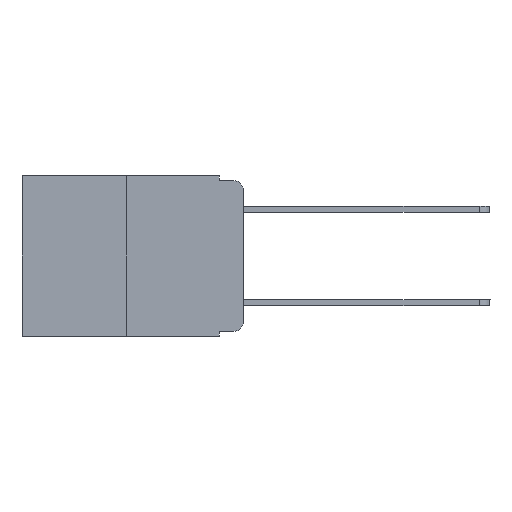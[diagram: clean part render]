
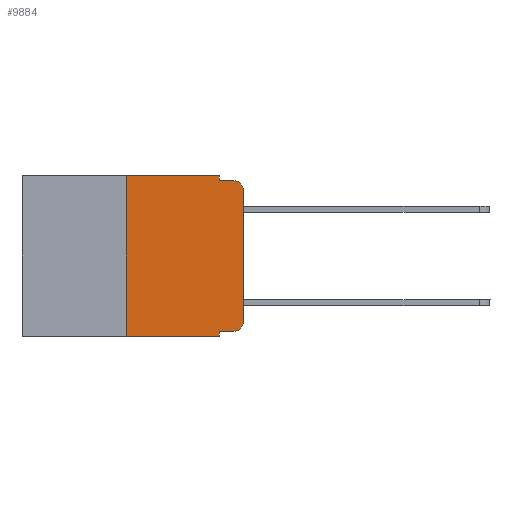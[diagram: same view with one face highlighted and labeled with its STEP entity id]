
A CAD part, left-side view. The second image highlights one B-rep face of the part: STEP entity #9884.
In plain terms, the highlighted planar face has unit normal (-1, 0, 0).
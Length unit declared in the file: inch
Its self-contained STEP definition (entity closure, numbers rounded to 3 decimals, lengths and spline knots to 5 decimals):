
#197 = DIRECTION ( 'NONE',  ( 0., -1., 0. ) ) ;
#403 = LINE ( 'NONE', #5945, #8011 ) ;
#513 = DIRECTION ( 'NONE',  ( 0., -1., 0. ) ) ;
#864 = VERTEX_POINT ( 'NONE', #8967 ) ;
#872 = EDGE_LOOP ( 'NONE', ( #10765, #11012, #3093, #997, #9420, #1775, #10407, #6484, #1513, #9154 ) ) ;
#997 = ORIENTED_EDGE ( 'NONE', *, *, #5999, .F. ) ;
#1007 = CARTESIAN_POINT ( 'NONE',  ( 0., 0.473, 0. ) ) ;
#1102 = EDGE_CURVE ( 'NONE', #2378, #2417, #6632, .T. ) ;
#1237 = CARTESIAN_POINT ( 'NONE',  ( 0., 0.25, -0.343 ) ) ;
#1356 = CARTESIAN_POINT ( 'NONE',  ( 0., 0.473, -0.343 ) ) ;
#1513 = ORIENTED_EDGE ( 'NONE', *, *, #3057, .T. ) ;
#1562 = DIRECTION ( 'NONE',  ( -1., 0., 0. ) ) ;
#1775 = ORIENTED_EDGE ( 'NONE', *, *, #5760, .F. ) ;
#1803 = CARTESIAN_POINT ( 'NONE',  ( 0., 0., -0.313 ) ) ;
#2030 = CARTESIAN_POINT ( 'NONE',  ( 0., 0., 0. ) ) ;
#2205 = EDGE_CURVE ( 'NONE', #4691, #2378, #4605, .T. ) ;
#2235 = VERTEX_POINT ( 'NONE', #1237 ) ;
#2378 = VERTEX_POINT ( 'NONE', #6835 ) ;
#2417 = VERTEX_POINT ( 'NONE', #5220 ) ;
#2481 = DIRECTION ( 'NONE',  ( 0., 0., -1. ) ) ;
#2568 = EDGE_CURVE ( 'NONE', #10823, #3773, #5002, .T. ) ;
#2684 = DIRECTION ( 'NONE',  ( 1., 0., 0. ) ) ;
#2881 = VECTOR ( 'NONE', #8968, 39.37008 ) ;
#2986 = CARTESIAN_POINT ( 'NONE',  ( 0., 0.051, -0.333 ) ) ;
#3057 = EDGE_CURVE ( 'NONE', #10823, #3672, #9598, .T. ) ;
#3093 = ORIENTED_EDGE ( 'NONE', *, *, #5106, .F. ) ;
#3416 = DIRECTION ( 'NONE',  ( 0., 0., -1. ) ) ;
#3422 = FACE_OUTER_BOUND ( 'NONE', #872, .T. ) ;
#3605 = AXIS2_PLACEMENT_3D ( 'NONE', #7185, #4580, #6220 ) ;
#3672 = VERTEX_POINT ( 'NONE', #8116 ) ;
#3773 = VERTEX_POINT ( 'NONE', #4777 ) ;
#4003 = LINE ( 'NONE', #4593, #4669 ) ;
#4103 = DIRECTION ( 'NONE',  ( 0., 0., 1. ) ) ;
#4577 = CARTESIAN_POINT ( 'NONE',  ( 0., 0.25, 0. ) ) ;
#4580 = DIRECTION ( 'NONE',  ( -1., 0., 0. ) ) ;
#4593 = CARTESIAN_POINT ( 'NONE',  ( 0., 0.051, -0.01 ) ) ;
#4605 = LINE ( 'NONE', #2030, #2881 ) ;
#4624 = CARTESIAN_POINT ( 'NONE',  ( 0., 0.051, -0.333 ) ) ;
#4669 = VECTOR ( 'NONE', #8872, 39.37008 ) ;
#4691 = VERTEX_POINT ( 'NONE', #1803 ) ;
#4745 = VECTOR ( 'NONE', #9021, 39.37008 ) ;
#4777 = CARTESIAN_POINT ( 'NONE',  ( 0., 0.051, -0.343 ) ) ;
#5002 = LINE ( 'NONE', #10677, #4745 ) ;
#5106 = EDGE_CURVE ( 'NONE', #864, #2417, #4003, .T. ) ;
#5220 = CARTESIAN_POINT ( 'NONE',  ( 0., 0.02, -0.01 ) ) ;
#5339 = VERTEX_POINT ( 'NONE', #5754 ) ;
#5754 = CARTESIAN_POINT ( 'NONE',  ( 0., 0.051, 0. ) ) ;
#5760 = EDGE_CURVE ( 'NONE', #2235, #9523, #11060, .T. ) ;
#5945 = CARTESIAN_POINT ( 'NONE',  ( 0., 0.051, 0. ) ) ;
#5970 = CARTESIAN_POINT ( 'NONE',  ( 0., 0.02, -0.313 ) ) ;
#5999 = EDGE_CURVE ( 'NONE', #5339, #864, #403, .T. ) ;
#6049 = PLANE ( 'NONE',  #7792 ) ;
#6220 = DIRECTION ( 'NONE',  ( 0., 0., -1. ) ) ;
#6411 = CIRCLE ( 'NONE', #6960, 0.02 ) ;
#6484 = ORIENTED_EDGE ( 'NONE', *, *, #2568, .F. ) ;
#6621 = CARTESIAN_POINT ( 'NONE',  ( 0., 0.25, 0. ) ) ;
#6632 = CIRCLE ( 'NONE', #3605, 0.02 ) ;
#6732 = EDGE_CURVE ( 'NONE', #9523, #5339, #9863, .T. ) ;
#6835 = CARTESIAN_POINT ( 'NONE',  ( 0., 0., -0.03 ) ) ;
#6960 = AXIS2_PLACEMENT_3D ( 'NONE', #5970, #1562, #2481 ) ;
#7185 = CARTESIAN_POINT ( 'NONE',  ( 0., 0.02, -0.03 ) ) ;
#7750 = EDGE_CURVE ( 'NONE', #3672, #4691, #6411, .T. ) ;
#7792 = AXIS2_PLACEMENT_3D ( 'NONE', #10751, #2684, #8586 ) ;
#8011 = VECTOR ( 'NONE', #3416, 39.37008 ) ;
#8023 = EDGE_CURVE ( 'NONE', #2235, #3773, #8715, .T. ) ;
#8116 = CARTESIAN_POINT ( 'NONE',  ( 0., 0.02, -0.333 ) ) ;
#8586 = DIRECTION ( 'NONE',  ( 0., 0., -1. ) ) ;
#8715 = LINE ( 'NONE', #1356, #9965 ) ;
#8872 = DIRECTION ( 'NONE',  ( 0., -1., 0. ) ) ;
#8967 = CARTESIAN_POINT ( 'NONE',  ( 0., 0.051, -0.01 ) ) ;
#8968 = DIRECTION ( 'NONE',  ( 0., 0., 1. ) ) ;
#9021 = DIRECTION ( 'NONE',  ( 0., 0., -1. ) ) ;
#9154 = ORIENTED_EDGE ( 'NONE', *, *, #7750, .T. ) ;
#9420 = ORIENTED_EDGE ( 'NONE', *, *, #6732, .F. ) ;
#9523 = VERTEX_POINT ( 'NONE', #4577 ) ;
#9598 = LINE ( 'NONE', #2986, #11249 ) ;
#9830 = DIRECTION ( 'NONE',  ( 0., -1., 0. ) ) ;
#9863 = LINE ( 'NONE', #1007, #10400 ) ;
#9884 = ADVANCED_FACE ( 'NONE', ( #3422 ), #6049, .F. ) ;
#9965 = VECTOR ( 'NONE', #513, 39.37008 ) ;
#10400 = VECTOR ( 'NONE', #197, 39.37008 ) ;
#10407 = ORIENTED_EDGE ( 'NONE', *, *, #8023, .T. ) ;
#10677 = CARTESIAN_POINT ( 'NONE',  ( 0., 0.051, 0. ) ) ;
#10751 = CARTESIAN_POINT ( 'NONE',  ( 0., 0.473, 0. ) ) ;
#10765 = ORIENTED_EDGE ( 'NONE', *, *, #2205, .T. ) ;
#10823 = VERTEX_POINT ( 'NONE', #4624 ) ;
#10937 = VECTOR ( 'NONE', #4103, 39.37008 ) ;
#11012 = ORIENTED_EDGE ( 'NONE', *, *, #1102, .T. ) ;
#11060 = LINE ( 'NONE', #6621, #10937 ) ;
#11249 = VECTOR ( 'NONE', #9830, 39.37008 ) ;
